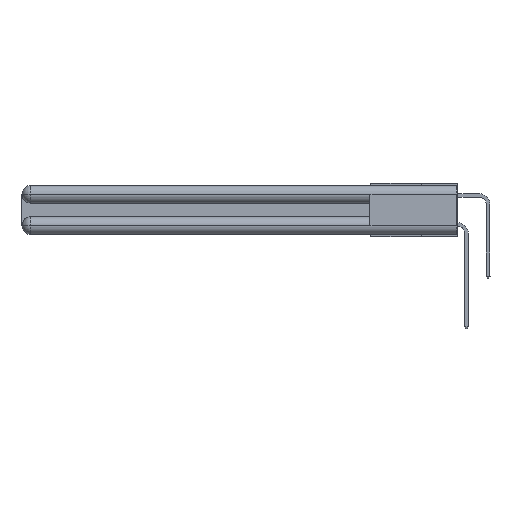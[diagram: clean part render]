
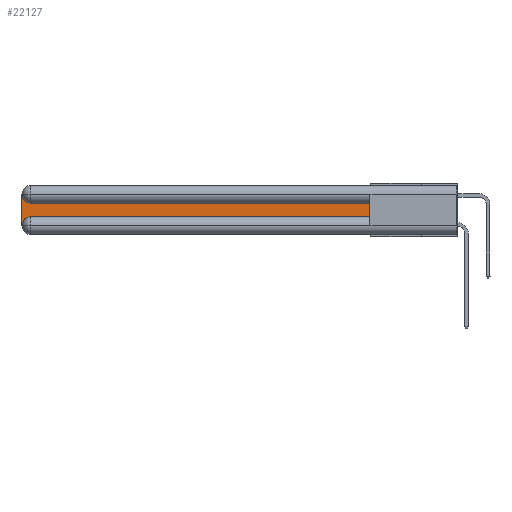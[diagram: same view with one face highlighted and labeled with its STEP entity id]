
A CAD part, left-side view. The second image highlights one B-rep face of the part: STEP entity #22127.
In plain terms, the highlighted planar face has unit normal (-1, 0, 0).
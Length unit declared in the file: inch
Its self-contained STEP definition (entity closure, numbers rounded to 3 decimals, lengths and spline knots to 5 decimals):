
#967 = EDGE_CURVE ( 'NONE', #12229, #20268, #21565, .T. ) ;
#1488 = EDGE_CURVE ( 'NONE', #12184, #12229, #12487, .T. ) ;
#2191 = DIRECTION ( 'NONE',  ( 0., 0., 1. ) ) ;
#2427 = VERTEX_POINT ( 'NONE', #28060 ) ;
#2643 = CARTESIAN_POINT ( 'NONE',  ( 0.075, 2.94, -0.2175 ) ) ;
#2695 = AXIS2_PLACEMENT_3D ( 'NONE', #19082, #5816, #24359 ) ;
#4370 = LINE ( 'NONE', #27780, #8565 ) ;
#4936 = CARTESIAN_POINT ( 'NONE',  ( 0.075, 3., -0.1225 ) ) ;
#5816 = DIRECTION ( 'NONE',  ( 1., 0., 0. ) ) ;
#6486 = VERTEX_POINT ( 'NONE', #2643 ) ;
#6889 = AXIS2_PLACEMENT_3D ( 'NONE', #4936, #26041, #10218 ) ;
#7962 = EDGE_CURVE ( 'NONE', #2427, #6486, #16080, .T. ) ;
#8565 = VECTOR ( 'NONE', #33054, 39.37008 ) ;
#8593 = VECTOR ( 'NONE', #2191, 39.37008 ) ;
#9161 = EDGE_CURVE ( 'NONE', #20268, #2427, #22307, .T. ) ;
#9645 = DIRECTION ( 'NONE',  ( 0., 1., 0. ) ) ;
#10024 = CARTESIAN_POINT ( 'NONE',  ( 0.075, 2.94, -0.2775 ) ) ;
#10054 = CARTESIAN_POINT ( 'NONE',  ( 0.075, 0.6, -0.2175 ) ) ;
#10218 = DIRECTION ( 'NONE',  ( 0., 0., -1. ) ) ;
#10976 = ORIENTED_EDGE ( 'NONE', *, *, #18525, .T. ) ;
#11303 = CARTESIAN_POINT ( 'NONE',  ( 0.075, 3., -0.2175 ) ) ;
#11925 = ORIENTED_EDGE ( 'NONE', *, *, #967, .T. ) ;
#12184 = VERTEX_POINT ( 'NONE', #25358 ) ;
#12229 = VERTEX_POINT ( 'NONE', #18282 ) ;
#12487 = LINE ( 'NONE', #30588, #34016 ) ;
#12633 = AXIS2_PLACEMENT_3D ( 'NONE', #10024, #20456, #28526 ) ;
#12762 = PLANE ( 'NONE',  #6889 ) ;
#13287 = ORIENTED_EDGE ( 'NONE', *, *, #7962, .T. ) ;
#15315 = CARTESIAN_POINT ( 'NONE',  ( 0.075, 0.6, -0.2175 ) ) ;
#15848 = ORIENTED_EDGE ( 'NONE', *, *, #17836, .T. ) ;
#16080 = CIRCLE ( 'NONE', #12633, 0.06 ) ;
#17836 = EDGE_CURVE ( 'NONE', #20523, #12184, #23482, .T. ) ;
#18282 = CARTESIAN_POINT ( 'NONE',  ( 0.075, 2.94, -0.1225 ) ) ;
#18525 = EDGE_CURVE ( 'NONE', #6486, #20523, #4370, .T. ) ;
#19000 = FACE_OUTER_BOUND ( 'NONE', #21770, .T. ) ;
#19082 = CARTESIAN_POINT ( 'NONE',  ( 0.075, 2.94, -0.0625 ) ) ;
#20268 = VERTEX_POINT ( 'NONE', #29382 ) ;
#20456 = DIRECTION ( 'NONE',  ( 1., 0., 0. ) ) ;
#20523 = VERTEX_POINT ( 'NONE', #15315 ) ;
#21565 = CIRCLE ( 'NONE', #2695, 0.06 ) ;
#21770 = EDGE_LOOP ( 'NONE', ( #33661, #11925, #34300, #13287, #10976, #15848 ) ) ;
#22127 = ADVANCED_FACE ( 'NONE', ( #19000 ), #12762, .F. ) ;
#22307 = LINE ( 'NONE', #11303, #23130 ) ;
#23130 = VECTOR ( 'NONE', #32857, 39.37008 ) ;
#23482 = LINE ( 'NONE', #10054, #8593 ) ;
#24359 = DIRECTION ( 'NONE',  ( 0., 0., -1. ) ) ;
#25358 = CARTESIAN_POINT ( 'NONE',  ( 0.075, 0.6, -0.1225 ) ) ;
#26041 = DIRECTION ( 'NONE',  ( 1., 0., 0. ) ) ;
#27780 = CARTESIAN_POINT ( 'NONE',  ( 0.075, 0.6, -0.2175 ) ) ;
#28060 = CARTESIAN_POINT ( 'NONE',  ( 0.075, 3., -0.2775 ) ) ;
#28526 = DIRECTION ( 'NONE',  ( 0., 0., -1. ) ) ;
#29382 = CARTESIAN_POINT ( 'NONE',  ( 0.075, 3., -0.0625 ) ) ;
#30588 = CARTESIAN_POINT ( 'NONE',  ( 0.075, 0.6, -0.1225 ) ) ;
#32857 = DIRECTION ( 'NONE',  ( 0., 0., -1. ) ) ;
#33054 = DIRECTION ( 'NONE',  ( 0., -1., 0. ) ) ;
#33661 = ORIENTED_EDGE ( 'NONE', *, *, #1488, .T. ) ;
#34016 = VECTOR ( 'NONE', #9645, 39.37008 ) ;
#34300 = ORIENTED_EDGE ( 'NONE', *, *, #9161, .T. ) ;
